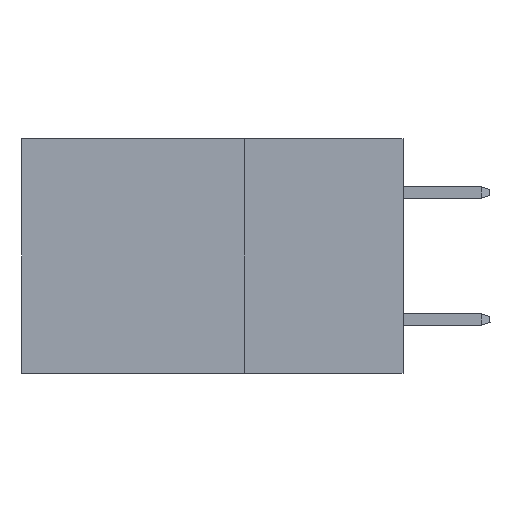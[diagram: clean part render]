
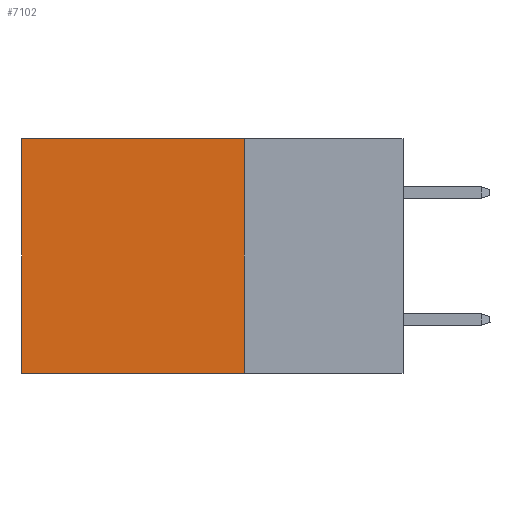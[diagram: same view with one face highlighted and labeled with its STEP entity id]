
A CAD part, left-side view. The second image highlights one B-rep face of the part: STEP entity #7102.
In plain terms, the highlighted planar face has unit normal (-1, 0, 0).
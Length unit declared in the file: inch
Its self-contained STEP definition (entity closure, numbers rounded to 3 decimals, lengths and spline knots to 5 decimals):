
#288 = LINE ( 'NONE', #14052, #4424 ) ;
#387 = EDGE_CURVE ( 'NONE', #3414, #6107, #14957, .T. ) ;
#721 = ORIENTED_EDGE ( 'NONE', *, *, #387, .T. ) ;
#1107 = ORIENTED_EDGE ( 'NONE', *, *, #16429, .T. ) ;
#1654 = DIRECTION ( 'NONE',  ( 0., 0., -1. ) ) ;
#1721 = DIRECTION ( 'NONE',  ( 0., 1., 0. ) ) ;
#1800 = CARTESIAN_POINT ( 'NONE',  ( 0.2875, 0.6, -0.37 ) ) ;
#1954 = CARTESIAN_POINT ( 'NONE',  ( 0.2875, 0.25, 0. ) ) ;
#1994 = AXIS2_PLACEMENT_3D ( 'NONE', #1954, #3325, #10780 ) ;
#3325 = DIRECTION ( 'NONE',  ( 1., 0., 0. ) ) ;
#3414 = VERTEX_POINT ( 'NONE', #8565 ) ;
#3595 = VECTOR ( 'NONE', #4738, 39.37008 ) ;
#3929 = CARTESIAN_POINT ( 'NONE',  ( 0.2875, 0.6, 0. ) ) ;
#4424 = VECTOR ( 'NONE', #1654, 39.37008 ) ;
#4738 = DIRECTION ( 'NONE',  ( 0., 1., 0. ) ) ;
#4801 = CARTESIAN_POINT ( 'NONE',  ( 0.2875, 0.6, 0. ) ) ;
#4934 = EDGE_CURVE ( 'NONE', #3414, #7476, #288, .T. ) ;
#6107 = VERTEX_POINT ( 'NONE', #4801 ) ;
#6634 = CARTESIAN_POINT ( 'NONE',  ( 0.2875, 0.25, -0.37 ) ) ;
#7102 = ADVANCED_FACE ( 'NONE', ( #14231 ), #20871, .F. ) ;
#7476 = VERTEX_POINT ( 'NONE', #6634 ) ;
#8565 = CARTESIAN_POINT ( 'NONE',  ( 0.2875, 0.25, 0. ) ) ;
#10477 = DIRECTION ( 'NONE',  ( 0., 0., -1. ) ) ;
#10780 = DIRECTION ( 'NONE',  ( 0., 0., -1. ) ) ;
#11681 = ORIENTED_EDGE ( 'NONE', *, *, #12844, .F. ) ;
#12668 = LINE ( 'NONE', #3929, #13318 ) ;
#12844 = EDGE_CURVE ( 'NONE', #7476, #17695, #14232, .T. ) ;
#13318 = VECTOR ( 'NONE', #10477, 39.37008 ) ;
#13369 = ORIENTED_EDGE ( 'NONE', *, *, #4934, .F. ) ;
#14052 = CARTESIAN_POINT ( 'NONE',  ( 0.2875, 0.25, 0. ) ) ;
#14231 = FACE_OUTER_BOUND ( 'NONE', #21535, .T. ) ;
#14232 = LINE ( 'NONE', #21219, #14651 ) ;
#14651 = VECTOR ( 'NONE', #1721, 39.37008 ) ;
#14957 = LINE ( 'NONE', #20445, #3595 ) ;
#16429 = EDGE_CURVE ( 'NONE', #6107, #17695, #12668, .T. ) ;
#17695 = VERTEX_POINT ( 'NONE', #1800 ) ;
#20445 = CARTESIAN_POINT ( 'NONE',  ( 0.2875, 0.25, 0. ) ) ;
#20871 = PLANE ( 'NONE',  #1994 ) ;
#21219 = CARTESIAN_POINT ( 'NONE',  ( 0.2875, 0.25, -0.37 ) ) ;
#21535 = EDGE_LOOP ( 'NONE', ( #1107, #11681, #13369, #721 ) ) ;
